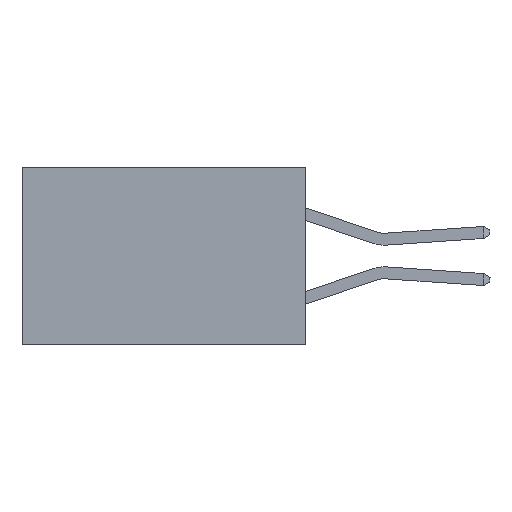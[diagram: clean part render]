
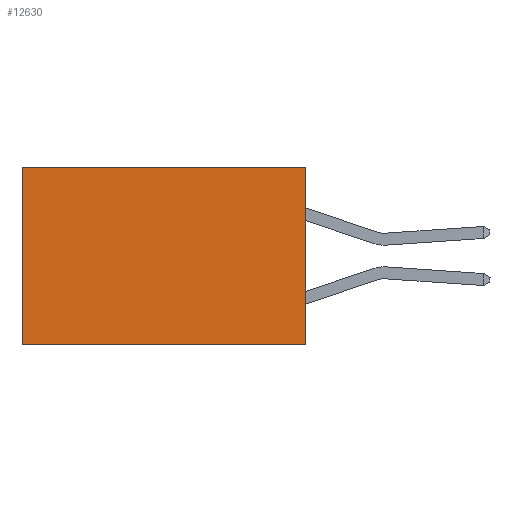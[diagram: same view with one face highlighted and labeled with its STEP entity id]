
A CAD part, left-side view. The second image highlights one B-rep face of the part: STEP entity #12630.
In plain terms, the highlighted planar face has unit normal (-1, 0, 0).
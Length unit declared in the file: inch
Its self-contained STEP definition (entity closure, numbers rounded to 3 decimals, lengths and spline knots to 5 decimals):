
#621 = CARTESIAN_POINT ( 'NONE',  ( 0.277, 0., -0.37 ) ) ;
#646 = LINE ( 'NONE', #4193, #8726 ) ;
#1720 = CARTESIAN_POINT ( 'NONE',  ( 0.277, 0., 0. ) ) ;
#2282 = CARTESIAN_POINT ( 'NONE',  ( 0.277, 0.59, 0. ) ) ;
#2386 = DIRECTION ( 'NONE',  ( 1., 0., 0. ) ) ;
#2472 = ORIENTED_EDGE ( 'NONE', *, *, #17525, .F. ) ;
#2838 = EDGE_LOOP ( 'NONE', ( #16498, #2472, #12778, #8900 ) ) ;
#3529 = DIRECTION ( 'NONE',  ( 0., 0., -1. ) ) ;
#3547 = VECTOR ( 'NONE', #20706, 39.37008 ) ;
#4193 = CARTESIAN_POINT ( 'NONE',  ( 0.277, 0.59, -0.37 ) ) ;
#4228 = CARTESIAN_POINT ( 'NONE',  ( 0.277, 0.59, -0.37 ) ) ;
#5369 = FACE_OUTER_BOUND ( 'NONE', #2838, .T. ) ;
#6516 = LINE ( 'NONE', #14125, #14744 ) ;
#7373 = EDGE_CURVE ( 'NONE', #13358, #8344, #646, .T. ) ;
#7535 = LINE ( 'NONE', #19050, #3547 ) ;
#7587 = DIRECTION ( 'NONE',  ( 0., 1., 0. ) ) ;
#8344 = VERTEX_POINT ( 'NONE', #4228 ) ;
#8726 = VECTOR ( 'NONE', #3529, 39.37008 ) ;
#8900 = ORIENTED_EDGE ( 'NONE', *, *, #16122, .T. ) ;
#10021 = CARTESIAN_POINT ( 'NONE',  ( 0.277, 0., -0.37 ) ) ;
#12496 = PLANE ( 'NONE',  #19199 ) ;
#12630 = ADVANCED_FACE ( 'NONE', ( #5369 ), #12496, .F. ) ;
#12778 = ORIENTED_EDGE ( 'NONE', *, *, #20790, .F. ) ;
#13005 = VERTEX_POINT ( 'NONE', #10021 ) ;
#13358 = VERTEX_POINT ( 'NONE', #2282 ) ;
#14125 = CARTESIAN_POINT ( 'NONE',  ( 0.277, 0., -0.37 ) ) ;
#14138 = DIRECTION ( 'NONE',  ( 0., 0., -1. ) ) ;
#14299 = LINE ( 'NONE', #20810, #17051 ) ;
#14744 = VECTOR ( 'NONE', #7587, 39.37008 ) ;
#16122 = EDGE_CURVE ( 'NONE', #18899, #13358, #14299, .T. ) ;
#16498 = ORIENTED_EDGE ( 'NONE', *, *, #7373, .T. ) ;
#17051 = VECTOR ( 'NONE', #20881, 39.37008 ) ;
#17525 = EDGE_CURVE ( 'NONE', #13005, #8344, #6516, .T. ) ;
#18899 = VERTEX_POINT ( 'NONE', #1720 ) ;
#19050 = CARTESIAN_POINT ( 'NONE',  ( 0.277, 0., -0.37 ) ) ;
#19199 = AXIS2_PLACEMENT_3D ( 'NONE', #621, #2386, #14138 ) ;
#20706 = DIRECTION ( 'NONE',  ( 0., 0., -1. ) ) ;
#20790 = EDGE_CURVE ( 'NONE', #18899, #13005, #7535, .T. ) ;
#20810 = CARTESIAN_POINT ( 'NONE',  ( 0.277, 0., 0. ) ) ;
#20881 = DIRECTION ( 'NONE',  ( 0., 1., 0. ) ) ;
